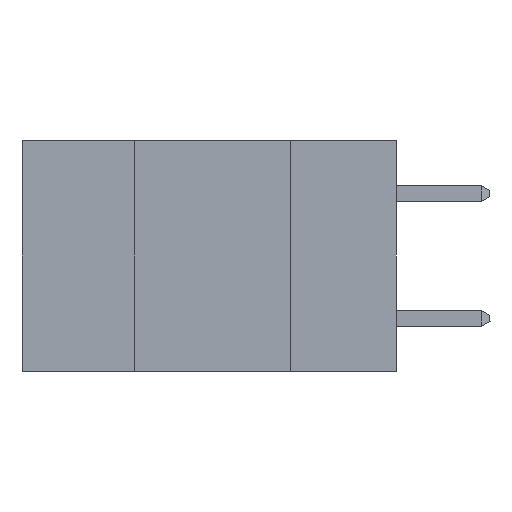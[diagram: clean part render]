
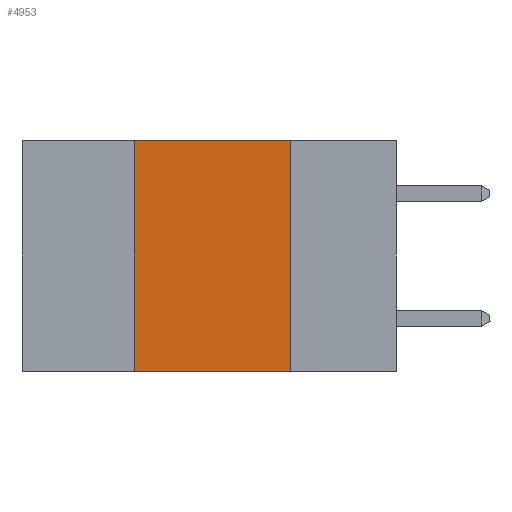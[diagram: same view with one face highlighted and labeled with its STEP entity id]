
A CAD part, left-side view. The second image highlights one B-rep face of the part: STEP entity #4953.
In plain terms, the highlighted planar face has unit normal (-1, 0, 0).
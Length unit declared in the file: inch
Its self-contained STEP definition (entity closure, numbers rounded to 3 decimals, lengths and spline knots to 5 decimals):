
#315 = VERTEX_POINT ( 'NONE', #20753 ) ;
#405 = DIRECTION ( 'NONE',  ( 0., 0., -1. ) ) ;
#1575 = VERTEX_POINT ( 'NONE', #21308 ) ;
#2241 = ORIENTED_EDGE ( 'NONE', *, *, #10045, .F. ) ;
#3343 = DIRECTION ( 'NONE',  ( 0., 0., -1. ) ) ;
#3626 = AXIS2_PLACEMENT_3D ( 'NONE', #7516, #11341, #405 ) ;
#4322 = DIRECTION ( 'NONE',  ( 0., -1., 0. ) ) ;
#4697 = DIRECTION ( 'NONE',  ( 0., -1., 0. ) ) ;
#4953 = ADVANCED_FACE ( 'NONE', ( #22413 ), #22258, .F. ) ;
#4976 = LINE ( 'NONE', #15715, #14774 ) ;
#5892 = EDGE_CURVE ( 'NONE', #17490, #1575, #8028, .T. ) ;
#7450 = VECTOR ( 'NONE', #4322, 39.37008 ) ;
#7516 = CARTESIAN_POINT ( 'NONE',  ( 0., 0.6, 0. ) ) ;
#7978 = CARTESIAN_POINT ( 'NONE',  ( 0., 0.6, -0.37 ) ) ;
#8028 = LINE ( 'NONE', #7978, #7450 ) ;
#8433 = CARTESIAN_POINT ( 'NONE',  ( 0., 0.42, -0.37 ) ) ;
#8805 = EDGE_CURVE ( 'NONE', #17231, #1575, #13700, .T. ) ;
#9575 = CARTESIAN_POINT ( 'NONE',  ( 0., 0.17, 0. ) ) ;
#10045 = EDGE_CURVE ( 'NONE', #17490, #315, #20679, .T. ) ;
#10835 = ORIENTED_EDGE ( 'NONE', *, *, #8805, .F. ) ;
#10986 = VECTOR ( 'NONE', #16863, 39.37008 ) ;
#11341 = DIRECTION ( 'NONE',  ( 1., 0., 0. ) ) ;
#12505 = CARTESIAN_POINT ( 'NONE',  ( 0., 0.17, -0.37 ) ) ;
#13700 = LINE ( 'NONE', #12505, #18509 ) ;
#14774 = VECTOR ( 'NONE', #4697, 39.37008 ) ;
#15047 = CARTESIAN_POINT ( 'NONE',  ( 0., 0.42, -0.37 ) ) ;
#15467 = EDGE_CURVE ( 'NONE', #315, #17231, #4976, .T. ) ;
#15715 = CARTESIAN_POINT ( 'NONE',  ( 0., 0.6, 0. ) ) ;
#16863 = DIRECTION ( 'NONE',  ( 0., 0., 1. ) ) ;
#17231 = VERTEX_POINT ( 'NONE', #9575 ) ;
#17490 = VERTEX_POINT ( 'NONE', #8433 ) ;
#17921 = EDGE_LOOP ( 'NONE', ( #10835, #21099, #2241, #22254 ) ) ;
#18509 = VECTOR ( 'NONE', #3343, 39.37008 ) ;
#20679 = LINE ( 'NONE', #15047, #10986 ) ;
#20753 = CARTESIAN_POINT ( 'NONE',  ( 0., 0.42, 0. ) ) ;
#21099 = ORIENTED_EDGE ( 'NONE', *, *, #15467, .F. ) ;
#21308 = CARTESIAN_POINT ( 'NONE',  ( 0., 0.17, -0.37 ) ) ;
#22254 = ORIENTED_EDGE ( 'NONE', *, *, #5892, .T. ) ;
#22258 = PLANE ( 'NONE',  #3626 ) ;
#22413 = FACE_OUTER_BOUND ( 'NONE', #17921, .T. ) ;
